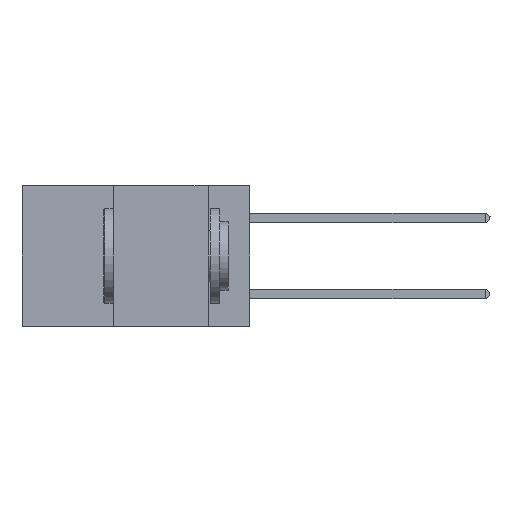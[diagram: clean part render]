
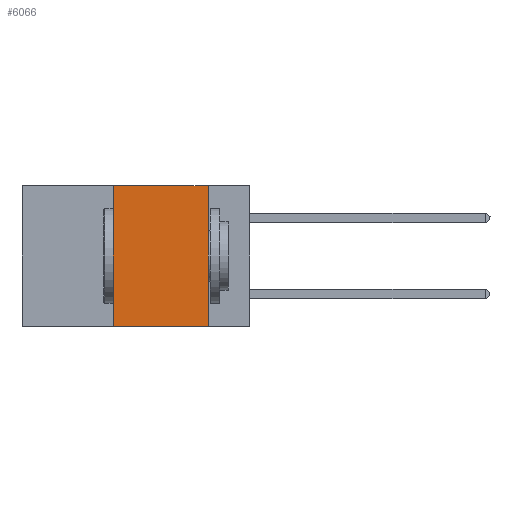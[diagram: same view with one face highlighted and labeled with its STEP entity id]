
A CAD part, left-side view. The second image highlights one B-rep face of the part: STEP entity #6066.
In plain terms, the highlighted planar face has unit normal (-1, 0, 0).
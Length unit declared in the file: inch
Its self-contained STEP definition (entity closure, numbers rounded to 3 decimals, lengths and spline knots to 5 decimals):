
#209 = FACE_OUTER_BOUND ( 'NONE', #16128, .T. ) ;
#945 = ORIENTED_EDGE ( 'NONE', *, *, #12466, .F. ) ;
#1414 = CARTESIAN_POINT ( 'NONE',  ( 0., 0.36, 0. ) ) ;
#2186 = VECTOR ( 'NONE', #23753, 39.37008 ) ;
#2627 = LINE ( 'NONE', #19644, #23218 ) ;
#2870 = EDGE_CURVE ( 'NONE', #3490, #15677, #21572, .T. ) ;
#3490 = VERTEX_POINT ( 'NONE', #6619 ) ;
#5317 = ORIENTED_EDGE ( 'NONE', *, *, #20028, .F. ) ;
#6066 = ADVANCED_FACE ( 'NONE', ( #209 ), #8336, .F. ) ;
#6619 = CARTESIAN_POINT ( 'NONE',  ( 0., 0.36, -0.37 ) ) ;
#7427 = CARTESIAN_POINT ( 'NONE',  ( 0., 0.11, -0.37 ) ) ;
#7805 = CARTESIAN_POINT ( 'NONE',  ( 0., 0.6, -0.37 ) ) ;
#8117 = VECTOR ( 'NONE', #9482, 39.37008 ) ;
#8336 = PLANE ( 'NONE',  #18838 ) ;
#9482 = DIRECTION ( 'NONE',  ( 0., -1., 0. ) ) ;
#9976 = LINE ( 'NONE', #21946, #14453 ) ;
#10613 = VERTEX_POINT ( 'NONE', #7427 ) ;
#10872 = CARTESIAN_POINT ( 'NONE',  ( 0., 0.11, 0. ) ) ;
#12466 = EDGE_CURVE ( 'NONE', #15677, #22222, #2627, .T. ) ;
#13476 = ORIENTED_EDGE ( 'NONE', *, *, #20993, .T. ) ;
#13767 = LINE ( 'NONE', #7805, #8117 ) ;
#13985 = CARTESIAN_POINT ( 'NONE',  ( 0., 0.6, 0. ) ) ;
#14453 = VECTOR ( 'NONE', #20021, 39.37008 ) ;
#15677 = VERTEX_POINT ( 'NONE', #1414 ) ;
#16128 = EDGE_LOOP ( 'NONE', ( #5317, #945, #21947, #13476 ) ) ;
#18838 = AXIS2_PLACEMENT_3D ( 'NONE', #13985, #23701, #21720 ) ;
#19644 = CARTESIAN_POINT ( 'NONE',  ( 0., 0.6, 0. ) ) ;
#20021 = DIRECTION ( 'NONE',  ( 0., 0., -1. ) ) ;
#20028 = EDGE_CURVE ( 'NONE', #22222, #10613, #9976, .T. ) ;
#20034 = CARTESIAN_POINT ( 'NONE',  ( 0., 0.36, 0. ) ) ;
#20993 = EDGE_CURVE ( 'NONE', #3490, #10613, #13767, .T. ) ;
#21572 = LINE ( 'NONE', #20034, #2186 ) ;
#21720 = DIRECTION ( 'NONE',  ( 0., 0., -1. ) ) ;
#21946 = CARTESIAN_POINT ( 'NONE',  ( 0., 0.11, 0. ) ) ;
#21947 = ORIENTED_EDGE ( 'NONE', *, *, #2870, .F. ) ;
#22222 = VERTEX_POINT ( 'NONE', #10872 ) ;
#22415 = DIRECTION ( 'NONE',  ( 0., -1., 0. ) ) ;
#23218 = VECTOR ( 'NONE', #22415, 39.37008 ) ;
#23701 = DIRECTION ( 'NONE',  ( 1., 0., 0. ) ) ;
#23753 = DIRECTION ( 'NONE',  ( 0., 0., 1. ) ) ;
